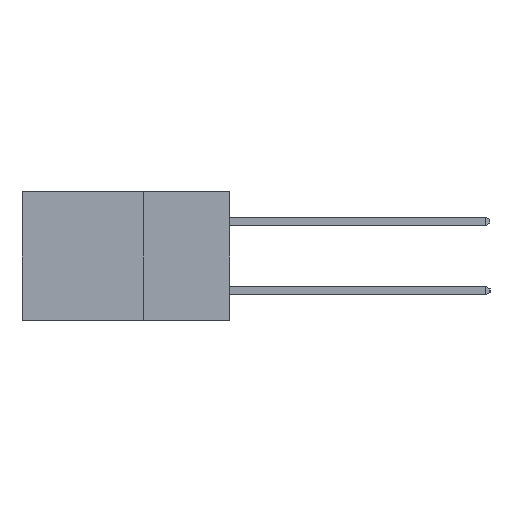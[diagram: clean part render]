
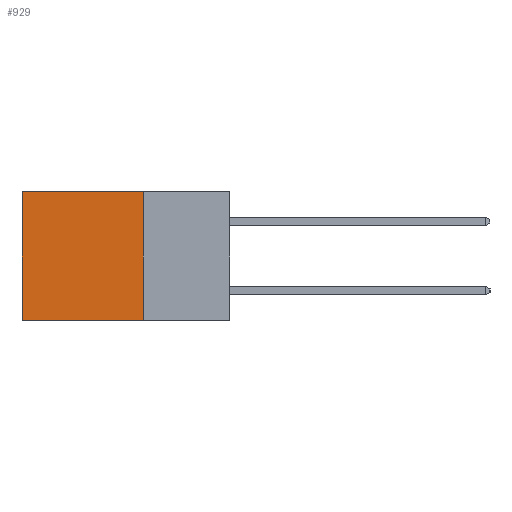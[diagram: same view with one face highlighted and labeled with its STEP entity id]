
A CAD part, left-side view. The second image highlights one B-rep face of the part: STEP entity #929.
In plain terms, the highlighted planar face has unit normal (-1, 0, 0).
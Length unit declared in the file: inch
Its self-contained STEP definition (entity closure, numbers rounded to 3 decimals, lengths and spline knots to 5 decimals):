
#628 = ORIENTED_EDGE ( 'NONE', *, *, #3767, .F. ) ;
#822 = LINE ( 'NONE', #24636, #20356 ) ;
#929 = ADVANCED_FACE ( 'NONE', ( #11257 ), #14952, .F. ) ;
#1418 = EDGE_CURVE ( 'NONE', #20283, #21041, #822, .T. ) ;
#2544 = VERTEX_POINT ( 'NONE', #11914 ) ;
#2562 = CARTESIAN_POINT ( 'NONE',  ( 0.2615, 0.25, -0.37 ) ) ;
#3048 = ORIENTED_EDGE ( 'NONE', *, *, #8254, .F. ) ;
#3767 = EDGE_CURVE ( 'NONE', #7382, #2544, #16484, .T. ) ;
#5908 = ORIENTED_EDGE ( 'NONE', *, *, #13537, .T. ) ;
#7253 = DIRECTION ( 'NONE',  ( 0., 1., 0. ) ) ;
#7382 = VERTEX_POINT ( 'NONE', #19755 ) ;
#8254 = EDGE_CURVE ( 'NONE', #20283, #7382, #21959, .T. ) ;
#10871 = AXIS2_PLACEMENT_3D ( 'NONE', #15310, #14949, #14925 ) ;
#11065 = DIRECTION ( 'NONE',  ( 0., 0., -1. ) ) ;
#11257 = FACE_OUTER_BOUND ( 'NONE', #11781, .T. ) ;
#11662 = VECTOR ( 'NONE', #14298, 39.37008 ) ;
#11781 = EDGE_LOOP ( 'NONE', ( #5908, #628, #3048, #13684 ) ) ;
#11914 = CARTESIAN_POINT ( 'NONE',  ( 0.2615, 0.6, -0.37 ) ) ;
#13537 = EDGE_CURVE ( 'NONE', #21041, #2544, #18823, .T. ) ;
#13684 = ORIENTED_EDGE ( 'NONE', *, *, #1418, .T. ) ;
#14298 = DIRECTION ( 'NONE',  ( 0., 0., -1. ) ) ;
#14925 = DIRECTION ( 'NONE',  ( 0., 0., -1. ) ) ;
#14949 = DIRECTION ( 'NONE',  ( 1., 0., 0. ) ) ;
#14952 = PLANE ( 'NONE',  #10871 ) ;
#15310 = CARTESIAN_POINT ( 'NONE',  ( 0.2615, 0.25, -0.37 ) ) ;
#15879 = VECTOR ( 'NONE', #7253, 39.37008 ) ;
#16484 = LINE ( 'NONE', #18970, #15879 ) ;
#18823 = LINE ( 'NONE', #24593, #24503 ) ;
#18970 = CARTESIAN_POINT ( 'NONE',  ( 0.2615, 0.25, -0.37 ) ) ;
#19755 = CARTESIAN_POINT ( 'NONE',  ( 0.2615, 0.25, -0.37 ) ) ;
#20283 = VERTEX_POINT ( 'NONE', #24777 ) ;
#20356 = VECTOR ( 'NONE', #24498, 39.37008 ) ;
#21041 = VERTEX_POINT ( 'NONE', #21156 ) ;
#21156 = CARTESIAN_POINT ( 'NONE',  ( 0.2615, 0.6, 0. ) ) ;
#21959 = LINE ( 'NONE', #2562, #11662 ) ;
#24498 = DIRECTION ( 'NONE',  ( 0., 1., 0. ) ) ;
#24503 = VECTOR ( 'NONE', #11065, 39.37008 ) ;
#24593 = CARTESIAN_POINT ( 'NONE',  ( 0.2615, 0.6, -0.37 ) ) ;
#24636 = CARTESIAN_POINT ( 'NONE',  ( 0.2615, 0.25, 0. ) ) ;
#24777 = CARTESIAN_POINT ( 'NONE',  ( 0.2615, 0.25, 0. ) ) ;
